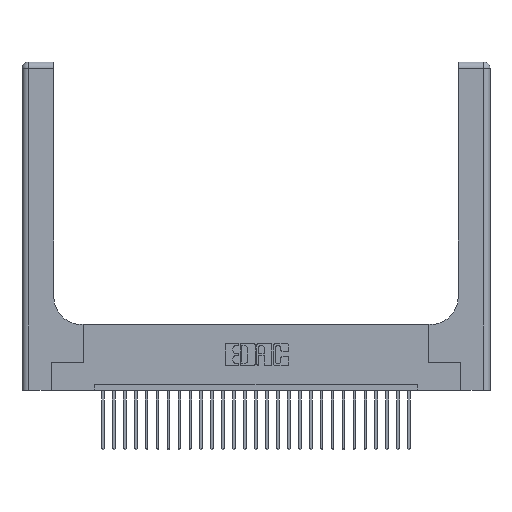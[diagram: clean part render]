
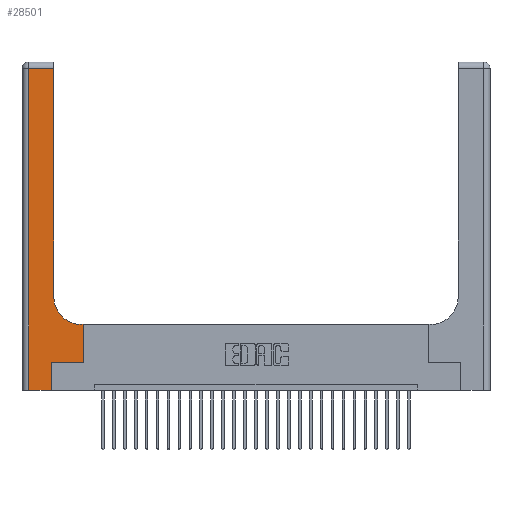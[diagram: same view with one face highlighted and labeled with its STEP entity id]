
A CAD part, top view. The second image highlights one B-rep face of the part: STEP entity #28501.
In plain terms, the highlighted planar face has unit normal (0, 0, 1).
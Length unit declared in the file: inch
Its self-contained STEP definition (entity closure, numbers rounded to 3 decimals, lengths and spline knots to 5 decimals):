
#54 = CARTESIAN_POINT ( 'NONE',  ( 0.269, 0., 0.37 ) ) ;
#513 = VECTOR ( 'NONE', #21578, 39.37008 ) ;
#699 = AXIS2_PLACEMENT_3D ( 'NONE', #11335, #13352, #13539 ) ;
#965 = EDGE_LOOP ( 'NONE', ( #2355, #2513, #8193, #26154, #5739, #15465, #11850, #11657, #14529 ) ) ;
#1428 = VERTEX_POINT ( 'NONE', #8386 ) ;
#1658 = DIRECTION ( 'NONE',  ( 1., 0., 0. ) ) ;
#1675 = AXIS2_PLACEMENT_3D ( 'NONE', #14876, #3878, #7914 ) ;
#2104 = VECTOR ( 'NONE', #15297, 39.37008 ) ;
#2355 = ORIENTED_EDGE ( 'NONE', *, *, #20237, .T. ) ;
#2450 = EDGE_CURVE ( 'NONE', #13441, #8241, #11062, .T. ) ;
#2513 = ORIENTED_EDGE ( 'NONE', *, *, #24429, .T. ) ;
#2545 = VECTOR ( 'NONE', #22315, 39.37008 ) ;
#3579 = VECTOR ( 'NONE', #22384, 39.37008 ) ;
#3878 = DIRECTION ( 'NONE',  ( 0., 0., -1. ) ) ;
#3944 = CARTESIAN_POINT ( 'NONE',  ( 0.5585, 0.25, 0.37 ) ) ;
#4105 = EDGE_CURVE ( 'NONE', #17542, #11950, #19305, .T. ) ;
#4671 = CARTESIAN_POINT ( 'NONE',  ( 0., 2.94, 0.37 ) ) ;
#5739 = ORIENTED_EDGE ( 'NONE', *, *, #14219, .T. ) ;
#6043 = VERTEX_POINT ( 'NONE', #12594 ) ;
#6949 = CARTESIAN_POINT ( 'NONE',  ( 0.5585, 0.25, 0.37 ) ) ;
#7155 = DIRECTION ( 'NONE',  ( -1., 0., 0. ) ) ;
#7914 = DIRECTION ( 'NONE',  ( 1., 0., 0. ) ) ;
#8068 = VECTOR ( 'NONE', #1658, 39.37008 ) ;
#8193 = ORIENTED_EDGE ( 'NONE', *, *, #2450, .T. ) ;
#8241 = VERTEX_POINT ( 'NONE', #22273 ) ;
#8386 = CARTESIAN_POINT ( 'NONE',  ( 0.269, 0.25, 0.37 ) ) ;
#8587 = DIRECTION ( 'NONE',  ( 0., 1., 0. ) ) ;
#8747 = CARTESIAN_POINT ( 'NONE',  ( 0.269, 0., 0.37 ) ) ;
#8794 = EDGE_CURVE ( 'NONE', #8241, #26944, #16872, .T. ) ;
#9108 = CARTESIAN_POINT ( 'NONE',  ( 0.06, 2.94, 0.37 ) ) ;
#10089 = EDGE_CURVE ( 'NONE', #12076, #27346, #20053, .T. ) ;
#11062 = LINE ( 'NONE', #20091, #16621 ) ;
#11335 = CARTESIAN_POINT ( 'NONE',  ( 0., 3., 0.37 ) ) ;
#11657 = ORIENTED_EDGE ( 'NONE', *, *, #11736, .T. ) ;
#11736 = EDGE_CURVE ( 'NONE', #11950, #12076, #17976, .T. ) ;
#11850 = ORIENTED_EDGE ( 'NONE', *, *, #4105, .T. ) ;
#11950 = VERTEX_POINT ( 'NONE', #19325 ) ;
#12076 = VERTEX_POINT ( 'NONE', #28487 ) ;
#12594 = CARTESIAN_POINT ( 'NONE',  ( 0.2915, 2.94, 0.37 ) ) ;
#12705 = VECTOR ( 'NONE', #7155, 39.37008 ) ;
#13352 = DIRECTION ( 'NONE',  ( 0., 0., -1. ) ) ;
#13441 = VERTEX_POINT ( 'NONE', #9108 ) ;
#13539 = DIRECTION ( 'NONE',  ( -1., 0., 0. ) ) ;
#14219 = EDGE_CURVE ( 'NONE', #26944, #1428, #25171, .T. ) ;
#14529 = ORIENTED_EDGE ( 'NONE', *, *, #10089, .T. ) ;
#14876 = CARTESIAN_POINT ( 'NONE',  ( 0.5415, 0.85, 0.37 ) ) ;
#14909 = CARTESIAN_POINT ( 'NONE',  ( 0.269, 0.25, 0.37 ) ) ;
#15297 = DIRECTION ( 'NONE',  ( 0., 1., 0. ) ) ;
#15465 = ORIENTED_EDGE ( 'NONE', *, *, #24658, .T. ) ;
#15491 = CARTESIAN_POINT ( 'NONE',  ( 0.2915, 0.6, 0.37 ) ) ;
#16621 = VECTOR ( 'NONE', #22304, 39.37008 ) ;
#16872 = LINE ( 'NONE', #25847, #513 ) ;
#17532 = VECTOR ( 'NONE', #8587, 39.37008 ) ;
#17542 = VERTEX_POINT ( 'NONE', #6949 ) ;
#17976 = LINE ( 'NONE', #15491, #12705 ) ;
#19017 = FACE_OUTER_BOUND ( 'NONE', #965, .T. ) ;
#19305 = LINE ( 'NONE', #3944, #17532 ) ;
#19325 = CARTESIAN_POINT ( 'NONE',  ( 0.5585, 0.6, 0.37 ) ) ;
#19936 = LINE ( 'NONE', #14909, #8068 ) ;
#20053 = CIRCLE ( 'NONE', #1675, 0.25 ) ;
#20091 = CARTESIAN_POINT ( 'NONE',  ( 0.06, 3., 0.37 ) ) ;
#20237 = EDGE_CURVE ( 'NONE', #27346, #6043, #27781, .T. ) ;
#21312 = LINE ( 'NONE', #4671, #3579 ) ;
#21578 = DIRECTION ( 'NONE',  ( 1., 0., 0. ) ) ;
#22273 = CARTESIAN_POINT ( 'NONE',  ( 0.06, 0., 0.37 ) ) ;
#22304 = DIRECTION ( 'NONE',  ( 0., -1., 0. ) ) ;
#22315 = DIRECTION ( 'NONE',  ( 0., 1., 0. ) ) ;
#22384 = DIRECTION ( 'NONE',  ( -1., 0., 0. ) ) ;
#22445 = PLANE ( 'NONE',  #699 ) ;
#24429 = EDGE_CURVE ( 'NONE', #6043, #13441, #21312, .T. ) ;
#24658 = EDGE_CURVE ( 'NONE', #1428, #17542, #19936, .T. ) ;
#25171 = LINE ( 'NONE', #54, #2545 ) ;
#25847 = CARTESIAN_POINT ( 'NONE',  ( 0., 0., 0.37 ) ) ;
#26154 = ORIENTED_EDGE ( 'NONE', *, *, #8794, .T. ) ;
#26944 = VERTEX_POINT ( 'NONE', #8747 ) ;
#27346 = VERTEX_POINT ( 'NONE', #27820 ) ;
#27781 = LINE ( 'NONE', #28322, #2104 ) ;
#27820 = CARTESIAN_POINT ( 'NONE',  ( 0.2915, 0.85, 0.37 ) ) ;
#28322 = CARTESIAN_POINT ( 'NONE',  ( 0.2915, 3., 0.37 ) ) ;
#28487 = CARTESIAN_POINT ( 'NONE',  ( 0.5415, 0.6, 0.37 ) ) ;
#28501 = ADVANCED_FACE ( 'NONE', ( #19017 ), #22445, .F. ) ;
